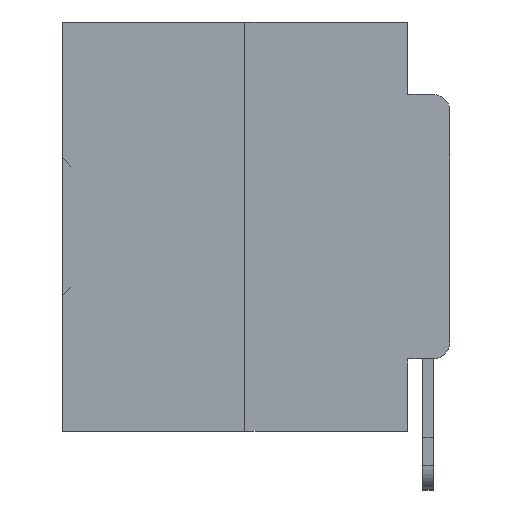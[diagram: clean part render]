
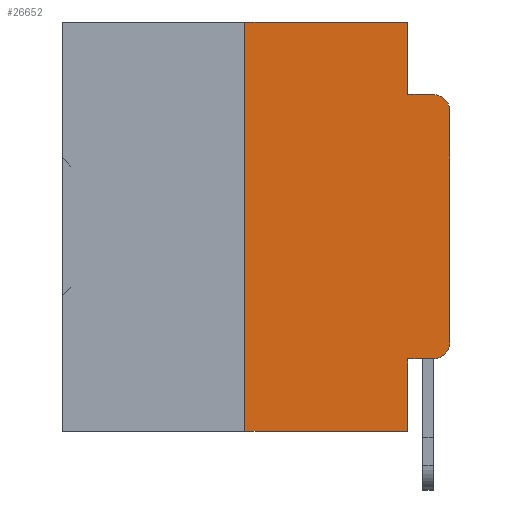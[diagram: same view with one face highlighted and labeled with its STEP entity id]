
A CAD part, left-side view. The second image highlights one B-rep face of the part: STEP entity #26652.
In plain terms, the highlighted planar face has unit normal (-1, 0, 0).
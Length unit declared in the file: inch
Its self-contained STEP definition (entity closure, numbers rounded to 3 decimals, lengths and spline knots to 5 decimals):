
#517 = ORIENTED_EDGE ( 'NONE', *, *, #24773, .T. ) ;
#1372 = VERTEX_POINT ( 'NONE', #14444 ) ;
#1393 = EDGE_CURVE ( 'NONE', #2951, #2623, #11306, .T. ) ;
#1746 = CARTESIAN_POINT ( 'NONE',  ( 0., 0.02, -0.0885 ) ) ;
#2012 = CARTESIAN_POINT ( 'NONE',  ( 0., 0.051, -0.0885 ) ) ;
#2152 = CARTESIAN_POINT ( 'NONE',  ( 0., 0.473, 0. ) ) ;
#2623 = VERTEX_POINT ( 'NONE', #26377 ) ;
#2900 = CARTESIAN_POINT ( 'NONE',  ( 0., 0.02, -0.3915 ) ) ;
#2914 = VECTOR ( 'NONE', #31214, 39.37008 ) ;
#2951 = VERTEX_POINT ( 'NONE', #24931 ) ;
#5149 = DIRECTION ( 'NONE',  ( 0., -1., 0. ) ) ;
#5306 = VECTOR ( 'NONE', #35487, 39.37008 ) ;
#5781 = VERTEX_POINT ( 'NONE', #34322 ) ;
#5945 = DIRECTION ( 'NONE',  ( 0., -1., 0. ) ) ;
#5977 = CARTESIAN_POINT ( 'NONE',  ( 0., 0.051, 0. ) ) ;
#6043 = DIRECTION ( 'NONE',  ( 0., 0., -1. ) ) ;
#6062 = VECTOR ( 'NONE', #5945, 39.37008 ) ;
#6131 = ORIENTED_EDGE ( 'NONE', *, *, #1393, .F. ) ;
#6429 = LINE ( 'NONE', #17626, #21693 ) ;
#6555 = CARTESIAN_POINT ( 'NONE',  ( 0., 0., -0.1085 ) ) ;
#6614 = VECTOR ( 'NONE', #36287, 39.37008 ) ;
#7683 = EDGE_CURVE ( 'NONE', #1372, #12591, #6429, .T. ) ;
#9580 = AXIS2_PLACEMENT_3D ( 'NONE', #2152, #38639, #20683 ) ;
#11306 = LINE ( 'NONE', #14574, #26492 ) ;
#11343 = CARTESIAN_POINT ( 'NONE',  ( 0., 0., 0. ) ) ;
#11581 = CARTESIAN_POINT ( 'NONE',  ( 0., 0., -0.3915 ) ) ;
#12265 = ORIENTED_EDGE ( 'NONE', *, *, #28763, .T. ) ;
#12591 = VERTEX_POINT ( 'NONE', #26787 ) ;
#13187 = CARTESIAN_POINT ( 'NONE',  ( 0., 0.02, -0.1085 ) ) ;
#13842 = EDGE_CURVE ( 'NONE', #1372, #14031, #14226, .T. ) ;
#14031 = VERTEX_POINT ( 'NONE', #33996 ) ;
#14172 = LINE ( 'NONE', #2012, #29268 ) ;
#14226 = LINE ( 'NONE', #33093, #6062 ) ;
#14444 = CARTESIAN_POINT ( 'NONE',  ( 0., 0.051, -0.4115 ) ) ;
#14574 = CARTESIAN_POINT ( 'NONE',  ( 0., 0.25, 0. ) ) ;
#14762 = LINE ( 'NONE', #5977, #6614 ) ;
#15215 = ORIENTED_EDGE ( 'NONE', *, *, #38794, .F. ) ;
#15898 = EDGE_CURVE ( 'NONE', #14031, #20697, #34770, .T. ) ;
#16085 = CARTESIAN_POINT ( 'NONE',  ( 0., 0.473, -0.5 ) ) ;
#16257 = DIRECTION ( 'NONE',  ( 0., 0., -1. ) ) ;
#16357 = EDGE_CURVE ( 'NONE', #2623, #31923, #27724, .T. ) ;
#16534 = VERTEX_POINT ( 'NONE', #6555 ) ;
#17617 = FACE_OUTER_BOUND ( 'NONE', #35896, .T. ) ;
#17626 = CARTESIAN_POINT ( 'NONE',  ( 0., 0.051, 0. ) ) ;
#17638 = PLANE ( 'NONE',  #9580 ) ;
#19006 = ORIENTED_EDGE ( 'NONE', *, *, #16357, .F. ) ;
#19048 = ORIENTED_EDGE ( 'NONE', *, *, #36290, .T. ) ;
#20188 = LINE ( 'NONE', #16085, #2914 ) ;
#20614 = AXIS2_PLACEMENT_3D ( 'NONE', #13187, #34269, #16257 ) ;
#20667 = DIRECTION ( 'NONE',  ( 0., 0., -1. ) ) ;
#20683 = DIRECTION ( 'NONE',  ( 0., 0., -1. ) ) ;
#20697 = VERTEX_POINT ( 'NONE', #11581 ) ;
#21693 = VECTOR ( 'NONE', #20667, 39.37008 ) ;
#24299 = DIRECTION ( 'NONE',  ( -1., 0., 0. ) ) ;
#24773 = EDGE_CURVE ( 'NONE', #20697, #16534, #29546, .T. ) ;
#24931 = CARTESIAN_POINT ( 'NONE',  ( 0., 0.25, -0.5 ) ) ;
#25089 = CARTESIAN_POINT ( 'NONE',  ( 0., 0.051, 0. ) ) ;
#26377 = CARTESIAN_POINT ( 'NONE',  ( 0., 0.25, 0. ) ) ;
#26492 = VECTOR ( 'NONE', #29606, 39.37008 ) ;
#26551 = VERTEX_POINT ( 'NONE', #1746 ) ;
#26652 = ADVANCED_FACE ( 'NONE', ( #17617 ), #17638, .F. ) ;
#26787 = CARTESIAN_POINT ( 'NONE',  ( 0., 0.051, -0.5 ) ) ;
#27724 = LINE ( 'NONE', #33025, #34736 ) ;
#28370 = ORIENTED_EDGE ( 'NONE', *, *, #32768, .F. ) ;
#28763 = EDGE_CURVE ( 'NONE', #16534, #26551, #35225, .T. ) ;
#29268 = VECTOR ( 'NONE', #5149, 39.37008 ) ;
#29546 = LINE ( 'NONE', #11343, #5306 ) ;
#29606 = DIRECTION ( 'NONE',  ( 0., 0., 1. ) ) ;
#30359 = ORIENTED_EDGE ( 'NONE', *, *, #13842, .T. ) ;
#31214 = DIRECTION ( 'NONE',  ( 0., -1., 0. ) ) ;
#31923 = VERTEX_POINT ( 'NONE', #25089 ) ;
#32768 = EDGE_CURVE ( 'NONE', #5781, #26551, #14172, .T. ) ;
#33025 = CARTESIAN_POINT ( 'NONE',  ( 0., 0.473, 0. ) ) ;
#33093 = CARTESIAN_POINT ( 'NONE',  ( 0., 0.051, -0.4115 ) ) ;
#33996 = CARTESIAN_POINT ( 'NONE',  ( 0., 0.02, -0.4115 ) ) ;
#34113 = ORIENTED_EDGE ( 'NONE', *, *, #15898, .T. ) ;
#34269 = DIRECTION ( 'NONE',  ( -1., 0., 0. ) ) ;
#34322 = CARTESIAN_POINT ( 'NONE',  ( 0., 0.051, -0.0885 ) ) ;
#34736 = VECTOR ( 'NONE', #35921, 39.37008 ) ;
#34770 = CIRCLE ( 'NONE', #36129, 0.02 ) ;
#35225 = CIRCLE ( 'NONE', #20614, 0.02 ) ;
#35487 = DIRECTION ( 'NONE',  ( 0., 0., 1. ) ) ;
#35896 = EDGE_LOOP ( 'NONE', ( #517, #12265, #28370, #15215, #19006, #6131, #19048, #36922, #30359, #34113 ) ) ;
#35921 = DIRECTION ( 'NONE',  ( 0., -1., 0. ) ) ;
#36129 = AXIS2_PLACEMENT_3D ( 'NONE', #2900, #24299, #6043 ) ;
#36287 = DIRECTION ( 'NONE',  ( 0., 0., -1. ) ) ;
#36290 = EDGE_CURVE ( 'NONE', #2951, #12591, #20188, .T. ) ;
#36922 = ORIENTED_EDGE ( 'NONE', *, *, #7683, .F. ) ;
#38639 = DIRECTION ( 'NONE',  ( 1., 0., 0. ) ) ;
#38794 = EDGE_CURVE ( 'NONE', #31923, #5781, #14762, .T. ) ;
